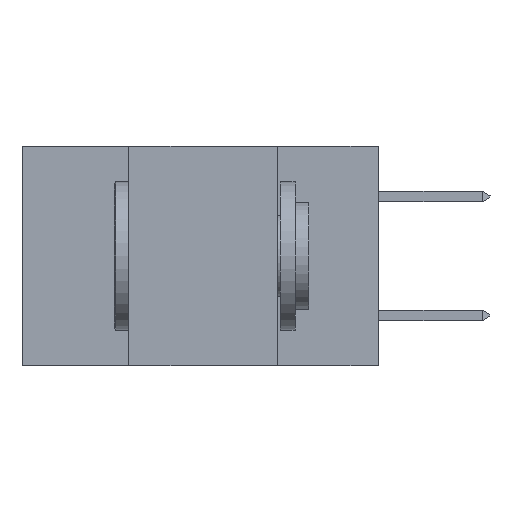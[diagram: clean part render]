
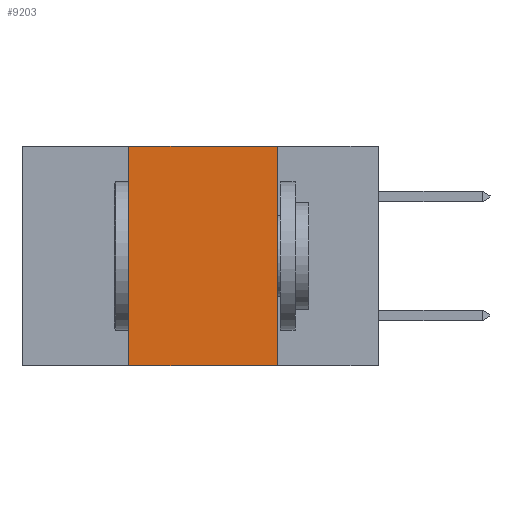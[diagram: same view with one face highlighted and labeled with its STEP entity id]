
A CAD part, left-side view. The second image highlights one B-rep face of the part: STEP entity #9203.
In plain terms, the highlighted planar face has unit normal (-1, 0, 0).
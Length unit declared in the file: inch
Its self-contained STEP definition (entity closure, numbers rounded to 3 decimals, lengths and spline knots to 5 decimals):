
#60 = CARTESIAN_POINT ( 'NONE',  ( 0., 0.42, -0.37 ) ) ;
#266 = ORIENTED_EDGE ( 'NONE', *, *, #5479, .F. ) ;
#977 = VERTEX_POINT ( 'NONE', #2960 ) ;
#1501 = LINE ( 'NONE', #7314, #4664 ) ;
#1735 = ORIENTED_EDGE ( 'NONE', *, *, #7570, .F. ) ;
#1851 = VERTEX_POINT ( 'NONE', #60 ) ;
#1905 = DIRECTION ( 'NONE',  ( 0., 0., -1. ) ) ;
#2512 = DIRECTION ( 'NONE',  ( 0., -1., 0. ) ) ;
#2632 = VERTEX_POINT ( 'NONE', #8085 ) ;
#2960 = CARTESIAN_POINT ( 'NONE',  ( 0., 0.17, 0. ) ) ;
#3328 = ORIENTED_EDGE ( 'NONE', *, *, #6937, .F. ) ;
#3510 = CARTESIAN_POINT ( 'NONE',  ( 0., 0.42, 0. ) ) ;
#3858 = EDGE_CURVE ( 'NONE', #1851, #2632, #8899, .T. ) ;
#4113 = VECTOR ( 'NONE', #2512, 39.37008 ) ;
#4271 = LINE ( 'NONE', #9197, #8722 ) ;
#4400 = CARTESIAN_POINT ( 'NONE',  ( 0., 0.42, -0.37 ) ) ;
#4664 = VECTOR ( 'NONE', #4792, 39.37008 ) ;
#4792 = DIRECTION ( 'NONE',  ( 0., -1., 0. ) ) ;
#5219 = DIRECTION ( 'NONE',  ( 0., 0., 1. ) ) ;
#5462 = CARTESIAN_POINT ( 'NONE',  ( 0., 0.6, 0. ) ) ;
#5479 = EDGE_CURVE ( 'NONE', #1851, #8544, #9276, .T. ) ;
#5514 = PLANE ( 'NONE',  #6188 ) ;
#6188 = AXIS2_PLACEMENT_3D ( 'NONE', #5462, #7723, #7134 ) ;
#6371 = EDGE_LOOP ( 'NONE', ( #1735, #3328, #266, #8535 ) ) ;
#6937 = EDGE_CURVE ( 'NONE', #8544, #977, #1501, .T. ) ;
#7134 = DIRECTION ( 'NONE',  ( 0., 0., -1. ) ) ;
#7314 = CARTESIAN_POINT ( 'NONE',  ( 0., 0.6, 0. ) ) ;
#7570 = EDGE_CURVE ( 'NONE', #977, #2632, #4271, .T. ) ;
#7723 = DIRECTION ( 'NONE',  ( 1., 0., 0. ) ) ;
#7934 = FACE_OUTER_BOUND ( 'NONE', #6371, .T. ) ;
#8085 = CARTESIAN_POINT ( 'NONE',  ( 0., 0.17, -0.37 ) ) ;
#8136 = CARTESIAN_POINT ( 'NONE',  ( 0., 0.6, -0.37 ) ) ;
#8535 = ORIENTED_EDGE ( 'NONE', *, *, #3858, .T. ) ;
#8544 = VERTEX_POINT ( 'NONE', #3510 ) ;
#8722 = VECTOR ( 'NONE', #1905, 39.37008 ) ;
#8727 = VECTOR ( 'NONE', #5219, 39.37008 ) ;
#8899 = LINE ( 'NONE', #8136, #4113 ) ;
#9197 = CARTESIAN_POINT ( 'NONE',  ( 0., 0.17, -0.37 ) ) ;
#9203 = ADVANCED_FACE ( 'NONE', ( #7934 ), #5514, .F. ) ;
#9276 = LINE ( 'NONE', #4400, #8727 ) ;
